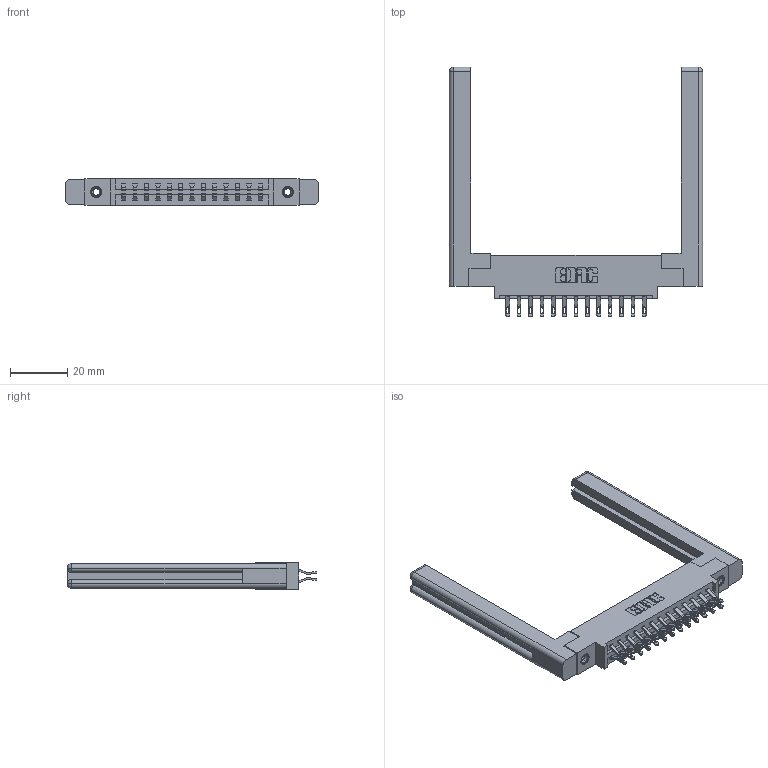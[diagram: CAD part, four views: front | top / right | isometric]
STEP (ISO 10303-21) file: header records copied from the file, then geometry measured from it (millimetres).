
FILE_DESCRIPTION (( 'STEP AP203' ), '1' );
FILE_NAME ('387-026-555-858.STEP', '2019-10-16T20:38:32', ( '' ), ( '' ), 'SwSTEP 2.0', 'SolidWorks 2016', '' );
FILE_SCHEMA (( 'CONFIG_CONTROL_DESIGN' ));
Length unit declared in the file: inch
Products named in the file (5): 307-220-058; 345-292-001_555 Tail; 387-026-555-858; 345-250-001_345-250-001-102; 337 Part_0.170 Offset - 0.156 Dia-TI
Assembly tree (31 placements, depth 2):
  387-026-555-858
    337 Part_0.170 Offset - 0.156 Dia-TI
    345-292-001_555 Tail  x26
    345-250-001_345-250-001-102  x2
    307-220-058  x2
Bounding box: 88.14 x 86.87 x 9.4 mm (x, y, z)
Volume: 16002.9 mm3; surface area: 15174 mm2
Topology: 31 solids, 31 shells, 1820 faces, 5591 edges, 3714 vertices
Faces by surface type: plane 1094, cylinder 702, cone 12, torus 12
Entity records: 16922 total; most frequent: CARTESIAN_POINT 2919, ORIENTED_EDGE 2764, DIRECTION 2522, EDGE_CURVE 1382, LINE 1186, VECTOR 1186, VERTEX_POINT 914, AXIS2_PLACEMENT_3D 668
